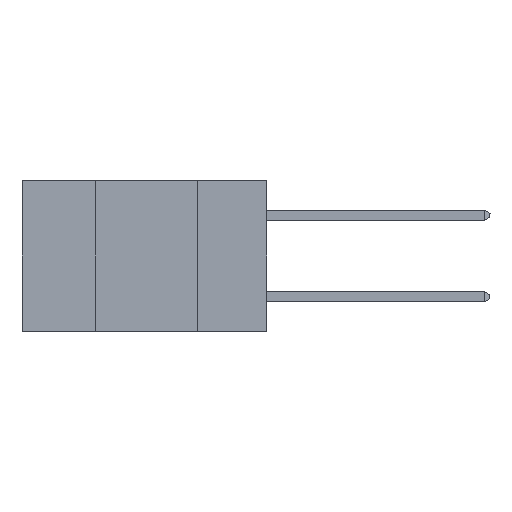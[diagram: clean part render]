
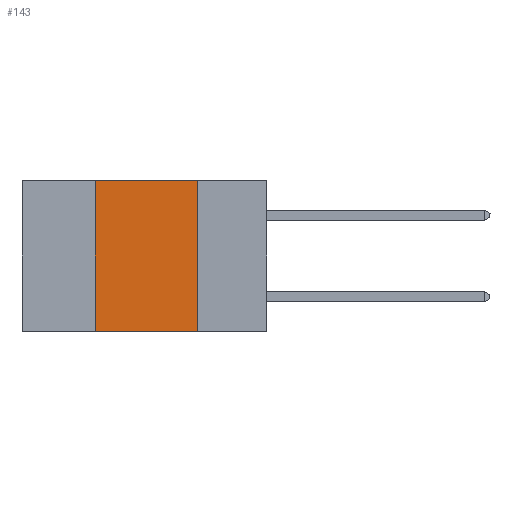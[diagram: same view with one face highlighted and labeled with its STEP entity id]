
A CAD part, left-side view. The second image highlights one B-rep face of the part: STEP entity #143.
In plain terms, the highlighted planar face has unit normal (-1, 0, 0).
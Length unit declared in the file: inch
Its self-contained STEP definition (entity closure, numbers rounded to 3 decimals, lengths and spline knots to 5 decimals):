
#143 = ADVANCED_FACE ( 'NONE', ( #9858 ), #7312, .F. ) ;
#359 = CARTESIAN_POINT ( 'NONE',  ( 0., 0.6, -0.37 ) ) ;
#457 = LINE ( 'NONE', #6084, #7721 ) ;
#556 = ORIENTED_EDGE ( 'NONE', *, *, #13542, .F. ) ;
#872 = VERTEX_POINT ( 'NONE', #13182 ) ;
#1169 = VECTOR ( 'NONE', #13866, 39.37008 ) ;
#1616 = LINE ( 'NONE', #12658, #1169 ) ;
#2228 = CARTESIAN_POINT ( 'NONE',  ( 0., 0.42, 0. ) ) ;
#6084 = CARTESIAN_POINT ( 'NONE',  ( 0., 0.17, 0. ) ) ;
#6566 = CARTESIAN_POINT ( 'NONE',  ( 0., 0.17, 0. ) ) ;
#7009 = ORIENTED_EDGE ( 'NONE', *, *, #15115, .F. ) ;
#7113 = VERTEX_POINT ( 'NONE', #6566 ) ;
#7312 = PLANE ( 'NONE',  #14767 ) ;
#7341 = EDGE_CURVE ( 'NONE', #13916, #8601, #8032, .T. ) ;
#7529 = LINE ( 'NONE', #359, #14022 ) ;
#7721 = VECTOR ( 'NONE', #14674, 39.37008 ) ;
#8032 = LINE ( 'NONE', #2228, #14149 ) ;
#8601 = VERTEX_POINT ( 'NONE', #9933 ) ;
#9292 = DIRECTION ( 'NONE',  ( 0., -1., 0. ) ) ;
#9858 = FACE_OUTER_BOUND ( 'NONE', #13318, .T. ) ;
#9933 = CARTESIAN_POINT ( 'NONE',  ( 0., 0.42, 0. ) ) ;
#10960 = DIRECTION ( 'NONE',  ( 0., 0., 1. ) ) ;
#12151 = CARTESIAN_POINT ( 'NONE',  ( 0., 0.42, -0.37 ) ) ;
#12658 = CARTESIAN_POINT ( 'NONE',  ( 0., 0.6, 0. ) ) ;
#13182 = CARTESIAN_POINT ( 'NONE',  ( 0., 0.17, -0.37 ) ) ;
#13318 = EDGE_LOOP ( 'NONE', ( #7009, #556, #14288, #15441 ) ) ;
#13542 = EDGE_CURVE ( 'NONE', #8601, #7113, #1616, .T. ) ;
#13866 = DIRECTION ( 'NONE',  ( 0., -1., 0. ) ) ;
#13916 = VERTEX_POINT ( 'NONE', #12151 ) ;
#14022 = VECTOR ( 'NONE', #9292, 39.37008 ) ;
#14149 = VECTOR ( 'NONE', #10960, 39.37008 ) ;
#14288 = ORIENTED_EDGE ( 'NONE', *, *, #7341, .F. ) ;
#14543 = DIRECTION ( 'NONE',  ( 1., 0., 0. ) ) ;
#14673 = DIRECTION ( 'NONE',  ( 0., 0., -1. ) ) ;
#14674 = DIRECTION ( 'NONE',  ( 0., 0., -1. ) ) ;
#14767 = AXIS2_PLACEMENT_3D ( 'NONE', #15060, #14543, #14673 ) ;
#14869 = EDGE_CURVE ( 'NONE', #13916, #872, #7529, .T. ) ;
#15060 = CARTESIAN_POINT ( 'NONE',  ( 0., 0.6, 0. ) ) ;
#15115 = EDGE_CURVE ( 'NONE', #7113, #872, #457, .T. ) ;
#15441 = ORIENTED_EDGE ( 'NONE', *, *, #14869, .T. ) ;
